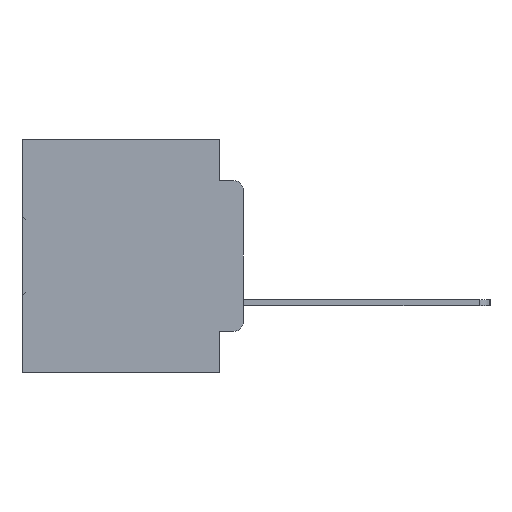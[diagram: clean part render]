
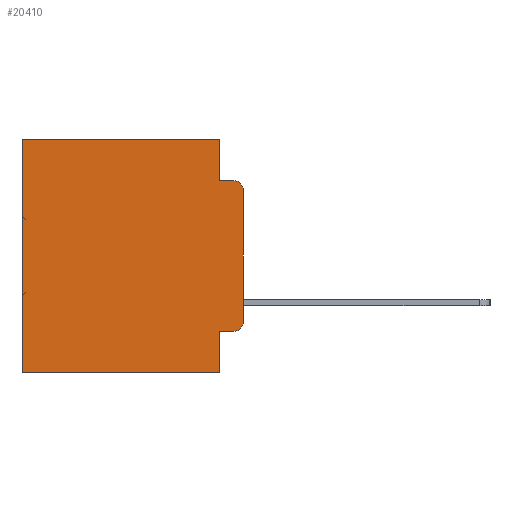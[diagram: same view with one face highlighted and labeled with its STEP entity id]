
A CAD part, left-side view. The second image highlights one B-rep face of the part: STEP entity #20410.
In plain terms, the highlighted planar face has unit normal (-1, 0, 0).
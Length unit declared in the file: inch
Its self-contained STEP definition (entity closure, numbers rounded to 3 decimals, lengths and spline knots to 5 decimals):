
#796 = VECTOR ( 'NONE', #20077, 39.37008 ) ;
#1155 = VECTOR ( 'NONE', #18790, 39.37008 ) ;
#1800 = EDGE_CURVE ( 'NONE', #32070, #35096, #32750, .T. ) ;
#2754 = CARTESIAN_POINT ( 'NONE',  ( 0.298, 0.051, 0. ) ) ;
#3443 = CARTESIAN_POINT ( 'NONE',  ( 0.298, 0.02, -0.4115 ) ) ;
#4040 = CARTESIAN_POINT ( 'NONE',  ( 0.298, 0.473, 0. ) ) ;
#4273 = CARTESIAN_POINT ( 'NONE',  ( 0.298, 0.02, -0.0885 ) ) ;
#4659 = VECTOR ( 'NONE', #8868, 39.37008 ) ;
#5688 = EDGE_CURVE ( 'NONE', #14251, #35096, #36396, .T. ) ;
#6814 = DIRECTION ( 'NONE',  ( 0., 0., -1. ) ) ;
#8111 = CARTESIAN_POINT ( 'NONE',  ( 0.298, 0.051, -0.0885 ) ) ;
#8129 = CARTESIAN_POINT ( 'NONE',  ( 0.298, 0.051, -0.0885 ) ) ;
#8479 = DIRECTION ( 'NONE',  ( 1., 0., 0. ) ) ;
#8748 = AXIS2_PLACEMENT_3D ( 'NONE', #30086, #13027, #32892 ) ;
#8868 = DIRECTION ( 'NONE',  ( 0., 0., -1. ) ) ;
#9411 = LINE ( 'NONE', #2754, #796 ) ;
#9550 = EDGE_CURVE ( 'NONE', #14251, #30173, #10682, .T. ) ;
#9786 = FACE_OUTER_BOUND ( 'NONE', #10578, .T. ) ;
#9841 = CARTESIAN_POINT ( 'NONE',  ( 0.298, 0.473, -0.5 ) ) ;
#10012 = AXIS2_PLACEMENT_3D ( 'NONE', #34200, #13354, #33293 ) ;
#10578 = EDGE_LOOP ( 'NONE', ( #28916, #36109, #18435, #22133, #36847, #34748, #13998, #15786, #25086, #11200 ) ) ;
#10682 = LINE ( 'NONE', #27227, #1155 ) ;
#11200 = ORIENTED_EDGE ( 'NONE', *, *, #23783, .T. ) ;
#11784 = CARTESIAN_POINT ( 'NONE',  ( 0.298, 0.051, 0. ) ) ;
#12382 = LINE ( 'NONE', #11784, #4659 ) ;
#12898 = LINE ( 'NONE', #20630, #27169 ) ;
#13027 = DIRECTION ( 'NONE',  ( -1., 0., 0. ) ) ;
#13341 = CARTESIAN_POINT ( 'NONE',  ( 0.298, 0.051, 0. ) ) ;
#13354 = DIRECTION ( 'NONE',  ( -1., 0., 0. ) ) ;
#13998 = ORIENTED_EDGE ( 'NONE', *, *, #31797, .F. ) ;
#14224 = LINE ( 'NONE', #18493, #22816 ) ;
#14251 = VERTEX_POINT ( 'NONE', #14508 ) ;
#14508 = CARTESIAN_POINT ( 'NONE',  ( 0.298, 0., -0.1085 ) ) ;
#14677 = VERTEX_POINT ( 'NONE', #13341 ) ;
#14930 = CARTESIAN_POINT ( 'NONE',  ( 0.298, 0.051, -0.5 ) ) ;
#15315 = VECTOR ( 'NONE', #24024, 39.37008 ) ;
#15331 = CARTESIAN_POINT ( 'NONE',  ( 0.298, 0., -0.5 ) ) ;
#15786 = ORIENTED_EDGE ( 'NONE', *, *, #29434, .F. ) ;
#17037 = CIRCLE ( 'NONE', #8748, 0.02 ) ;
#17192 = VERTEX_POINT ( 'NONE', #9841 ) ;
#18435 = ORIENTED_EDGE ( 'NONE', *, *, #1800, .F. ) ;
#18493 = CARTESIAN_POINT ( 'NONE',  ( 0.298, 0., 0. ) ) ;
#18790 = DIRECTION ( 'NONE',  ( 0., 0., -1. ) ) ;
#20077 = DIRECTION ( 'NONE',  ( 0., 0., -1. ) ) ;
#20410 = ADVANCED_FACE ( 'NONE', ( #9786 ), #34006, .F. ) ;
#20630 = CARTESIAN_POINT ( 'NONE',  ( 0.298, 0.051, -0.4115 ) ) ;
#20718 = VERTEX_POINT ( 'NONE', #26978 ) ;
#22133 = ORIENTED_EDGE ( 'NONE', *, *, #36875, .F. ) ;
#22689 = DIRECTION ( 'NONE',  ( 0., -1., 0. ) ) ;
#22816 = VECTOR ( 'NONE', #35382, 39.37008 ) ;
#23016 = LINE ( 'NONE', #15331, #15315 ) ;
#23551 = VECTOR ( 'NONE', #22689, 39.37008 ) ;
#23719 = VERTEX_POINT ( 'NONE', #32660 ) ;
#23783 = EDGE_CURVE ( 'NONE', #36418, #30173, #17037, .T. ) ;
#24024 = DIRECTION ( 'NONE',  ( 0., 1., 0. ) ) ;
#25086 = ORIENTED_EDGE ( 'NONE', *, *, #25641, .T. ) ;
#25641 = EDGE_CURVE ( 'NONE', #20718, #36418, #12898, .T. ) ;
#25660 = CARTESIAN_POINT ( 'NONE',  ( 0.298, 0., 0. ) ) ;
#26978 = CARTESIAN_POINT ( 'NONE',  ( 0.298, 0.051, -0.4115 ) ) ;
#27099 = VECTOR ( 'NONE', #6814, 39.37008 ) ;
#27169 = VECTOR ( 'NONE', #29135, 39.37008 ) ;
#27227 = CARTESIAN_POINT ( 'NONE',  ( 0.298, 0., 0. ) ) ;
#27997 = LINE ( 'NONE', #4040, #27099 ) ;
#28089 = AXIS2_PLACEMENT_3D ( 'NONE', #25660, #8479, #28514 ) ;
#28514 = DIRECTION ( 'NONE',  ( 0., 0., -1. ) ) ;
#28916 = ORIENTED_EDGE ( 'NONE', *, *, #9550, .F. ) ;
#29135 = DIRECTION ( 'NONE',  ( 0., -1., 0. ) ) ;
#29434 = EDGE_CURVE ( 'NONE', #20718, #32250, #9411, .T. ) ;
#30086 = CARTESIAN_POINT ( 'NONE',  ( 0.298, 0.02, -0.3915 ) ) ;
#30173 = VERTEX_POINT ( 'NONE', #35834 ) ;
#31797 = EDGE_CURVE ( 'NONE', #32250, #17192, #23016, .T. ) ;
#32070 = VERTEX_POINT ( 'NONE', #8129 ) ;
#32250 = VERTEX_POINT ( 'NONE', #14930 ) ;
#32660 = CARTESIAN_POINT ( 'NONE',  ( 0.298, 0.473, 0. ) ) ;
#32750 = LINE ( 'NONE', #8111, #23551 ) ;
#32892 = DIRECTION ( 'NONE',  ( 0., 0., -1. ) ) ;
#33293 = DIRECTION ( 'NONE',  ( 0., 0., -1. ) ) ;
#34006 = PLANE ( 'NONE',  #28089 ) ;
#34200 = CARTESIAN_POINT ( 'NONE',  ( 0.298, 0.02, -0.1085 ) ) ;
#34748 = ORIENTED_EDGE ( 'NONE', *, *, #35024, .T. ) ;
#35024 = EDGE_CURVE ( 'NONE', #23719, #17192, #27997, .T. ) ;
#35096 = VERTEX_POINT ( 'NONE', #4273 ) ;
#35382 = DIRECTION ( 'NONE',  ( 0., 1., 0. ) ) ;
#35834 = CARTESIAN_POINT ( 'NONE',  ( 0.298, 0., -0.3915 ) ) ;
#35969 = EDGE_CURVE ( 'NONE', #14677, #23719, #14224, .T. ) ;
#36109 = ORIENTED_EDGE ( 'NONE', *, *, #5688, .T. ) ;
#36396 = CIRCLE ( 'NONE', #10012, 0.02 ) ;
#36418 = VERTEX_POINT ( 'NONE', #3443 ) ;
#36847 = ORIENTED_EDGE ( 'NONE', *, *, #35969, .T. ) ;
#36875 = EDGE_CURVE ( 'NONE', #14677, #32070, #12382, .T. ) ;
